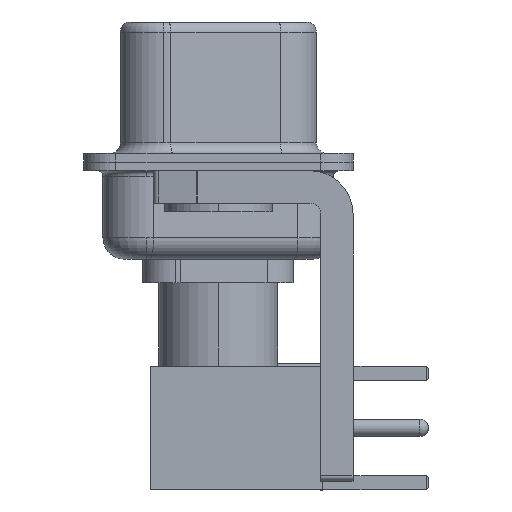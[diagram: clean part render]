
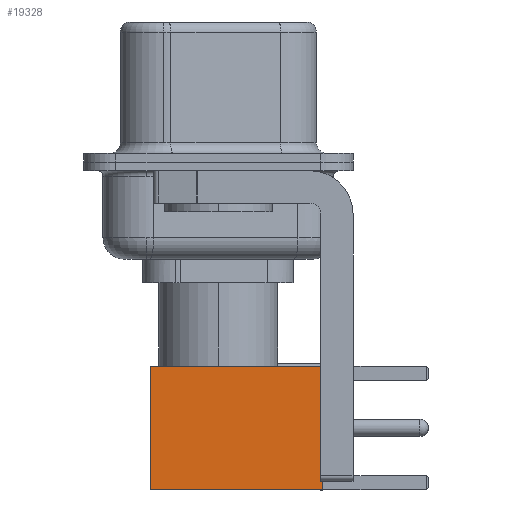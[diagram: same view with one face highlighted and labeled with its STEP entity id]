
A CAD part, left-side view. The second image highlights one B-rep face of the part: STEP entity #19328.
In plain terms, the highlighted face is planar.
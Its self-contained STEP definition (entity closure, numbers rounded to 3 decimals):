
#402 = EDGE_LOOP ( 'NONE', ( #1432, #28308, #4158, #6221 ) ) ;
#457 = VERTEX_POINT ( 'NONE', #27329 ) ;
#674 = DIRECTION ( 'NONE',  ( 0., 1., 0. ) ) ;
#829 = FACE_OUTER_BOUND ( 'NONE', #402, .T. ) ;
#835 = VERTEX_POINT ( 'NONE', #15895 ) ;
#1432 = ORIENTED_EDGE ( 'NONE', *, *, #29172, .T. ) ;
#2696 = CARTESIAN_POINT ( 'NONE',  ( 2.875, 2.875, 8. ) ) ;
#3443 = AXIS2_PLACEMENT_3D ( 'NONE', #28877, #674, #19520 ) ;
#4158 = ORIENTED_EDGE ( 'NONE', *, *, #24840, .F. ) ;
#6221 = ORIENTED_EDGE ( 'NONE', *, *, #19015, .F. ) ;
#8776 = CARTESIAN_POINT ( 'NONE',  ( 0., 2.875, 8. ) ) ;
#10708 = CARTESIAN_POINT ( 'NONE',  ( 0., 2.875, 0. ) ) ;
#11511 = LINE ( 'NONE', #12286, #21871 ) ;
#12286 = CARTESIAN_POINT ( 'NONE',  ( 2.875, 2.875, 0. ) ) ;
#12394 = VECTOR ( 'NONE', #18285, 1000. ) ;
#15535 = DIRECTION ( 'NONE',  ( -1., 0., 0. ) ) ;
#15895 = CARTESIAN_POINT ( 'NONE',  ( -2.875, 2.875, 8. ) ) ;
#17329 = CARTESIAN_POINT ( 'NONE',  ( -2.875, 2.875, 0. ) ) ;
#17731 = LINE ( 'NONE', #10708, #23889 ) ;
#18285 = DIRECTION ( 'NONE',  ( -1., 0., 0. ) ) ;
#19015 = EDGE_CURVE ( 'NONE', #24806, #835, #29834, .T. ) ;
#19315 = DIRECTION ( 'NONE',  ( 0., 0., -1. ) ) ;
#19328 = ADVANCED_FACE ( 'NONE', ( #829 ), #26401, .T. ) ;
#19517 = LINE ( 'NONE', #17329, #24534 ) ;
#19520 = DIRECTION ( 'NONE',  ( 0., 0., 1. ) ) ;
#21871 = VECTOR ( 'NONE', #19315, 1000. ) ;
#22552 = CARTESIAN_POINT ( 'NONE',  ( 2.875, 2.875, 0. ) ) ;
#23889 = VECTOR ( 'NONE', #15535, 1000. ) ;
#24534 = VECTOR ( 'NONE', #26856, 1000. ) ;
#24806 = VERTEX_POINT ( 'NONE', #2696 ) ;
#24840 = EDGE_CURVE ( 'NONE', #835, #457, #19517, .T. ) ;
#25917 = VERTEX_POINT ( 'NONE', #22552 ) ;
#26401 = PLANE ( 'NONE',  #3443 ) ;
#26856 = DIRECTION ( 'NONE',  ( 0., 0., -1. ) ) ;
#27329 = CARTESIAN_POINT ( 'NONE',  ( -2.875, 2.875, 0. ) ) ;
#28308 = ORIENTED_EDGE ( 'NONE', *, *, #29469, .T. ) ;
#28877 = CARTESIAN_POINT ( 'NONE',  ( 2.875, 2.875, 0. ) ) ;
#29172 = EDGE_CURVE ( 'NONE', #24806, #25917, #11511, .T. ) ;
#29469 = EDGE_CURVE ( 'NONE', #25917, #457, #17731, .T. ) ;
#29834 = LINE ( 'NONE', #8776, #12394 ) ;
